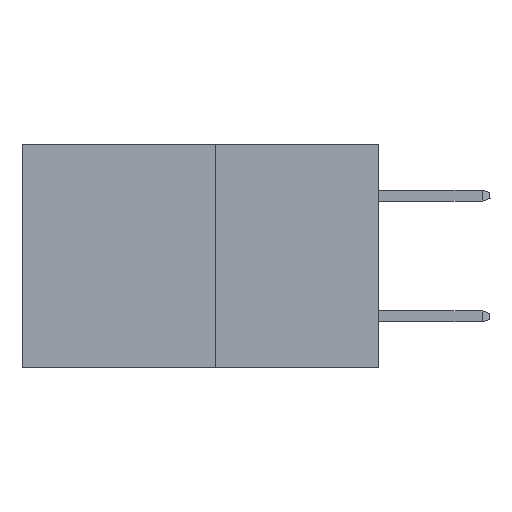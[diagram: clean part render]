
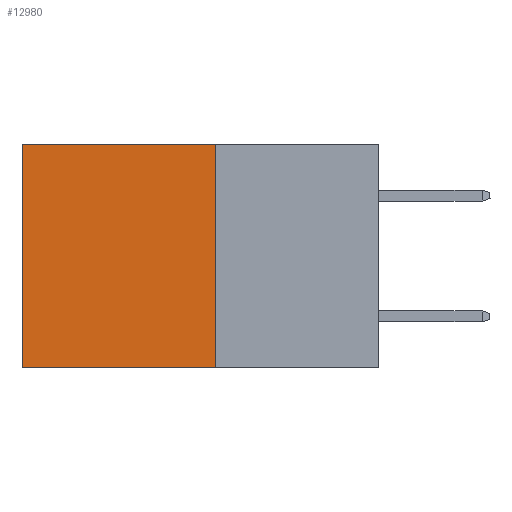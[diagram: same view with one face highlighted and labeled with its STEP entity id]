
A CAD part, left-side view. The second image highlights one B-rep face of the part: STEP entity #12980.
In plain terms, the highlighted planar face has unit normal (-1, 0, 0).
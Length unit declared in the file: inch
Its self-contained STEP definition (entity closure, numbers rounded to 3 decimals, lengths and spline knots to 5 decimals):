
#60 = ORIENTED_EDGE ( 'NONE', *, *, #15981, .T. ) ;
#1262 = VECTOR ( 'NONE', #2086, 39.37008 ) ;
#1310 = CARTESIAN_POINT ( 'NONE',  ( 0.277, 0.59, -0.37 ) ) ;
#2086 = DIRECTION ( 'NONE',  ( 0., 1., 0. ) ) ;
#2887 = DIRECTION ( 'NONE',  ( 0., 0., -1. ) ) ;
#3192 = EDGE_CURVE ( 'NONE', #7708, #4140, #11384, .T. ) ;
#3372 = CARTESIAN_POINT ( 'NONE',  ( 0.277, 0.27, -0.37 ) ) ;
#3928 = PLANE ( 'NONE',  #13465 ) ;
#4140 = VERTEX_POINT ( 'NONE', #10994 ) ;
#4258 = FACE_OUTER_BOUND ( 'NONE', #6540, .T. ) ;
#4346 = EDGE_CURVE ( 'NONE', #6029, #6122, #12848, .T. ) ;
#4929 = VECTOR ( 'NONE', #2887, 39.37008 ) ;
#6029 = VERTEX_POINT ( 'NONE', #11651 ) ;
#6122 = VERTEX_POINT ( 'NONE', #3372 ) ;
#6540 = EDGE_LOOP ( 'NONE', ( #8097, #16397, #11306, #60 ) ) ;
#6812 = DIRECTION ( 'NONE',  ( 0., 0., -1. ) ) ;
#7149 = VECTOR ( 'NONE', #13106, 39.37008 ) ;
#7708 = VERTEX_POINT ( 'NONE', #13390 ) ;
#7711 = EDGE_CURVE ( 'NONE', #6122, #4140, #13951, .T. ) ;
#7874 = DIRECTION ( 'NONE',  ( 1., 0., 0. ) ) ;
#8097 = ORIENTED_EDGE ( 'NONE', *, *, #3192, .T. ) ;
#8249 = LINE ( 'NONE', #8601, #1262 ) ;
#8601 = CARTESIAN_POINT ( 'NONE',  ( 0.277, 0.27, 0. ) ) ;
#10994 = CARTESIAN_POINT ( 'NONE',  ( 0.277, 0.59, -0.37 ) ) ;
#11306 = ORIENTED_EDGE ( 'NONE', *, *, #4346, .F. ) ;
#11384 = LINE ( 'NONE', #1310, #4929 ) ;
#11651 = CARTESIAN_POINT ( 'NONE',  ( 0.277, 0.27, 0. ) ) ;
#11799 = DIRECTION ( 'NONE',  ( 0., 0., -1. ) ) ;
#12458 = VECTOR ( 'NONE', #6812, 39.37008 ) ;
#12848 = LINE ( 'NONE', #14504, #12458 ) ;
#12980 = ADVANCED_FACE ( 'NONE', ( #4258 ), #3928, .F. ) ;
#13106 = DIRECTION ( 'NONE',  ( 0., 1., 0. ) ) ;
#13258 = CARTESIAN_POINT ( 'NONE',  ( 0.277, 0.27, -0.37 ) ) ;
#13390 = CARTESIAN_POINT ( 'NONE',  ( 0.277, 0.59, 0. ) ) ;
#13465 = AXIS2_PLACEMENT_3D ( 'NONE', #15479, #7874, #11799 ) ;
#13951 = LINE ( 'NONE', #13258, #7149 ) ;
#14504 = CARTESIAN_POINT ( 'NONE',  ( 0.277, 0.27, -0.37 ) ) ;
#15479 = CARTESIAN_POINT ( 'NONE',  ( 0.277, 0.27, -0.37 ) ) ;
#15981 = EDGE_CURVE ( 'NONE', #6029, #7708, #8249, .T. ) ;
#16397 = ORIENTED_EDGE ( 'NONE', *, *, #7711, .F. ) ;
